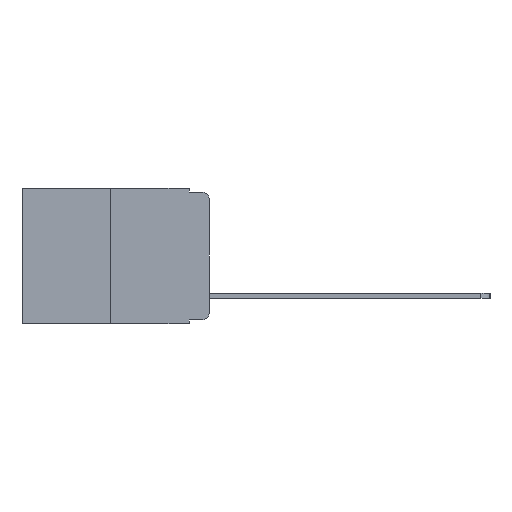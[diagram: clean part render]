
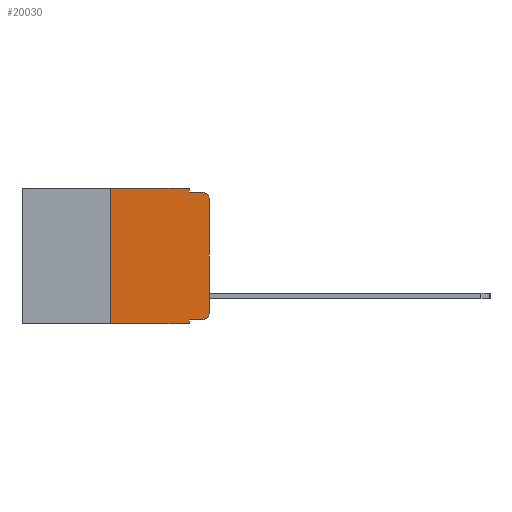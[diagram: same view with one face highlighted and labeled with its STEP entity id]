
A CAD part, left-side view. The second image highlights one B-rep face of the part: STEP entity #20030.
In plain terms, the highlighted planar face has unit normal (-1, 0, 0).
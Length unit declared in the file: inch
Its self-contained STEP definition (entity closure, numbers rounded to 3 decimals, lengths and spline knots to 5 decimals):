
#159 = CARTESIAN_POINT ( 'NONE',  ( 0., 0.051, 0. ) ) ;
#227 = DIRECTION ( 'NONE',  ( 0., -1., 0. ) ) ;
#272 = AXIS2_PLACEMENT_3D ( 'NONE', #5004, #20402, #9053 ) ;
#424 = ORIENTED_EDGE ( 'NONE', *, *, #15035, .T. ) ;
#466 = CARTESIAN_POINT ( 'NONE',  ( 0., 0., 0. ) ) ;
#666 = VERTEX_POINT ( 'NONE', #3398 ) ;
#714 = ORIENTED_EDGE ( 'NONE', *, *, #15816, .F. ) ;
#972 = VECTOR ( 'NONE', #5576, 39.37008 ) ;
#1159 = CARTESIAN_POINT ( 'NONE',  ( 0., 0.02, -0.01 ) ) ;
#1596 = EDGE_CURVE ( 'NONE', #21310, #12834, #9921, .T. ) ;
#1698 = DIRECTION ( 'NONE',  ( 0., 0., -1. ) ) ;
#1751 = VERTEX_POINT ( 'NONE', #17001 ) ;
#1762 = FACE_OUTER_BOUND ( 'NONE', #12886, .T. ) ;
#1965 = LINE ( 'NONE', #18528, #11711 ) ;
#2002 = LINE ( 'NONE', #159, #21742 ) ;
#2254 = ORIENTED_EDGE ( 'NONE', *, *, #3693, .T. ) ;
#2416 = EDGE_CURVE ( 'NONE', #16272, #5540, #22808, .T. ) ;
#2459 = EDGE_CURVE ( 'NONE', #19471, #1751, #2534, .T. ) ;
#2534 = LINE ( 'NONE', #17639, #16093 ) ;
#2751 = DIRECTION ( 'NONE',  ( 0., 0., 1. ) ) ;
#2877 = ORIENTED_EDGE ( 'NONE', *, *, #12033, .F. ) ;
#2986 = VECTOR ( 'NONE', #22470, 39.37008 ) ;
#2987 = CARTESIAN_POINT ( 'NONE',  ( 0., 0.051, -0.343 ) ) ;
#3242 = DIRECTION ( 'NONE',  ( 0., 0., -1. ) ) ;
#3398 = CARTESIAN_POINT ( 'NONE',  ( 0., 0.051, -0.01 ) ) ;
#3491 = CARTESIAN_POINT ( 'NONE',  ( 0., 0., -0.03 ) ) ;
#3693 = EDGE_CURVE ( 'NONE', #20946, #16272, #9240, .T. ) ;
#4625 = CARTESIAN_POINT ( 'NONE',  ( 0., 0.02, -0.333 ) ) ;
#4682 = VECTOR ( 'NONE', #12720, 39.37008 ) ;
#5004 = CARTESIAN_POINT ( 'NONE',  ( 0., 0.473, 0. ) ) ;
#5398 = CARTESIAN_POINT ( 'NONE',  ( 0., 0., -0.313 ) ) ;
#5540 = VERTEX_POINT ( 'NONE', #1159 ) ;
#5576 = DIRECTION ( 'NONE',  ( 0., 0., 1. ) ) ;
#5721 = VECTOR ( 'NONE', #22975, 39.37008 ) ;
#6068 = DIRECTION ( 'NONE',  ( 0., 0., -1. ) ) ;
#6418 = AXIS2_PLACEMENT_3D ( 'NONE', #24490, #13329, #1698 ) ;
#7153 = ORIENTED_EDGE ( 'NONE', *, *, #14304, .T. ) ;
#8075 = ORIENTED_EDGE ( 'NONE', *, *, #2459, .F. ) ;
#9053 = DIRECTION ( 'NONE',  ( 0., 0., -1. ) ) ;
#9240 = LINE ( 'NONE', #466, #23644 ) ;
#9446 = EDGE_CURVE ( 'NONE', #21310, #24388, #1965, .T. ) ;
#9607 = ORIENTED_EDGE ( 'NONE', *, *, #19612, .F. ) ;
#9921 = LINE ( 'NONE', #24416, #4682 ) ;
#10464 = CARTESIAN_POINT ( 'NONE',  ( 0., 0.051, -0.333 ) ) ;
#11273 = CARTESIAN_POINT ( 'NONE',  ( 0., 0.25, 0. ) ) ;
#11711 = VECTOR ( 'NONE', #3242, 39.37008 ) ;
#12033 = EDGE_CURVE ( 'NONE', #22003, #19471, #12540, .T. ) ;
#12358 = DIRECTION ( 'NONE',  ( 0., 0., -1. ) ) ;
#12540 = LINE ( 'NONE', #20872, #972 ) ;
#12720 = DIRECTION ( 'NONE',  ( 0., -1., 0. ) ) ;
#12834 = VERTEX_POINT ( 'NONE', #4625 ) ;
#12886 = EDGE_LOOP ( 'NONE', ( #2254, #19957, #9607, #714, #8075, #2877, #7153, #15607, #15282, #424 ) ) ;
#12961 = DIRECTION ( 'NONE',  ( -1., 0., 0. ) ) ;
#13329 = DIRECTION ( 'NONE',  ( -1., 0., 0. ) ) ;
#14304 = EDGE_CURVE ( 'NONE', #22003, #24388, #23236, .T. ) ;
#14575 = CARTESIAN_POINT ( 'NONE',  ( 0., 0.02, -0.03 ) ) ;
#15035 = EDGE_CURVE ( 'NONE', #12834, #20946, #21785, .T. ) ;
#15282 = ORIENTED_EDGE ( 'NONE', *, *, #1596, .T. ) ;
#15607 = ORIENTED_EDGE ( 'NONE', *, *, #9446, .F. ) ;
#15809 = AXIS2_PLACEMENT_3D ( 'NONE', #14575, #12961, #12358 ) ;
#15816 = EDGE_CURVE ( 'NONE', #1751, #666, #2002, .T. ) ;
#16093 = VECTOR ( 'NONE', #227, 39.37008 ) ;
#16207 = CARTESIAN_POINT ( 'NONE',  ( 0., 0.25, -0.343 ) ) ;
#16272 = VERTEX_POINT ( 'NONE', #3491 ) ;
#17001 = CARTESIAN_POINT ( 'NONE',  ( 0., 0.051, 0. ) ) ;
#17149 = LINE ( 'NONE', #21161, #5721 ) ;
#17639 = CARTESIAN_POINT ( 'NONE',  ( 0., 0.473, 0. ) ) ;
#18514 = PLANE ( 'NONE',  #272 ) ;
#18528 = CARTESIAN_POINT ( 'NONE',  ( 0., 0.051, 0. ) ) ;
#19471 = VERTEX_POINT ( 'NONE', #11273 ) ;
#19612 = EDGE_CURVE ( 'NONE', #666, #5540, #17149, .T. ) ;
#19957 = ORIENTED_EDGE ( 'NONE', *, *, #2416, .T. ) ;
#20030 = ADVANCED_FACE ( 'NONE', ( #1762 ), #18514, .F. ) ;
#20402 = DIRECTION ( 'NONE',  ( 1., 0., 0. ) ) ;
#20627 = CARTESIAN_POINT ( 'NONE',  ( 0., 0.473, -0.343 ) ) ;
#20872 = CARTESIAN_POINT ( 'NONE',  ( 0., 0.25, 0. ) ) ;
#20946 = VERTEX_POINT ( 'NONE', #5398 ) ;
#21161 = CARTESIAN_POINT ( 'NONE',  ( 0., 0.051, -0.01 ) ) ;
#21310 = VERTEX_POINT ( 'NONE', #10464 ) ;
#21742 = VECTOR ( 'NONE', #6068, 39.37008 ) ;
#21785 = CIRCLE ( 'NONE', #6418, 0.02 ) ;
#22003 = VERTEX_POINT ( 'NONE', #16207 ) ;
#22470 = DIRECTION ( 'NONE',  ( 0., -1., 0. ) ) ;
#22808 = CIRCLE ( 'NONE', #15809, 0.02 ) ;
#22975 = DIRECTION ( 'NONE',  ( 0., -1., 0. ) ) ;
#23236 = LINE ( 'NONE', #20627, #2986 ) ;
#23644 = VECTOR ( 'NONE', #2751, 39.37008 ) ;
#24388 = VERTEX_POINT ( 'NONE', #2987 ) ;
#24416 = CARTESIAN_POINT ( 'NONE',  ( 0., 0.051, -0.333 ) ) ;
#24490 = CARTESIAN_POINT ( 'NONE',  ( 0., 0.02, -0.313 ) ) ;
